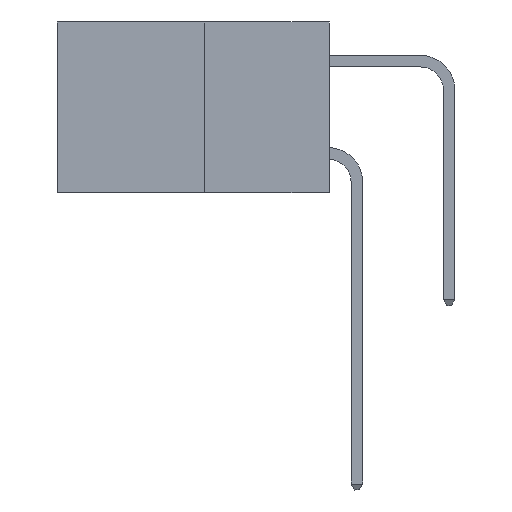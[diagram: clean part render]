
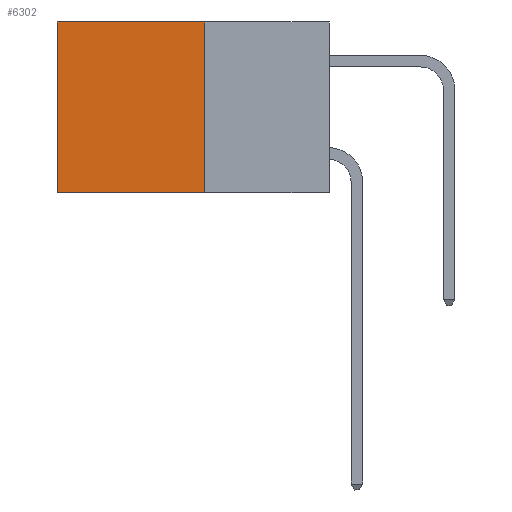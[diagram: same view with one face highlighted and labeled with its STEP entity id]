
A CAD part, left-side view. The second image highlights one B-rep face of the part: STEP entity #6302.
In plain terms, the highlighted planar face has unit normal (-1, 0, 0).
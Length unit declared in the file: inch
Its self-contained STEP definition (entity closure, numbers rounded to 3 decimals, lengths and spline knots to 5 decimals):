
#212 = CARTESIAN_POINT ( 'NONE',  ( 0.277, 0.27, -0.37 ) ) ;
#411 = DIRECTION ( 'NONE',  ( 0., 1., 0. ) ) ;
#683 = EDGE_LOOP ( 'NONE', ( #1466, #6687, #11780, #5957 ) ) ;
#749 = EDGE_CURVE ( 'NONE', #5637, #7984, #4505, .T. ) ;
#1007 = DIRECTION ( 'NONE',  ( 0., 0., -1. ) ) ;
#1109 = PLANE ( 'NONE',  #3783 ) ;
#1119 = EDGE_CURVE ( 'NONE', #7984, #6527, #11834, .T. ) ;
#1147 = DIRECTION ( 'NONE',  ( 1., 0., 0. ) ) ;
#1211 = DIRECTION ( 'NONE',  ( 0., 0., -1. ) ) ;
#1228 = CARTESIAN_POINT ( 'NONE',  ( 0.277, 0.27, -0.37 ) ) ;
#1466 = ORIENTED_EDGE ( 'NONE', *, *, #1119, .T. ) ;
#1794 = CARTESIAN_POINT ( 'NONE',  ( 0.277, 0.27, -0.37 ) ) ;
#1911 = DIRECTION ( 'NONE',  ( 0., 1., 0. ) ) ;
#2962 = CARTESIAN_POINT ( 'NONE',  ( 0.277, 0.27, 0. ) ) ;
#3019 = CARTESIAN_POINT ( 'NONE',  ( 0.277, 0.27, -0.37 ) ) ;
#3783 = AXIS2_PLACEMENT_3D ( 'NONE', #1794, #1147, #1007 ) ;
#4505 = LINE ( 'NONE', #8646, #9306 ) ;
#4783 = VECTOR ( 'NONE', #10424, 39.37008 ) ;
#5637 = VERTEX_POINT ( 'NONE', #2962 ) ;
#5957 = ORIENTED_EDGE ( 'NONE', *, *, #749, .T. ) ;
#5963 = EDGE_CURVE ( 'NONE', #8189, #6527, #12203, .T. ) ;
#6240 = FACE_OUTER_BOUND ( 'NONE', #683, .T. ) ;
#6280 = CARTESIAN_POINT ( 'NONE',  ( 0.277, 0.59, -0.37 ) ) ;
#6302 = ADVANCED_FACE ( 'NONE', ( #6240 ), #1109, .F. ) ;
#6527 = VERTEX_POINT ( 'NONE', #9547 ) ;
#6628 = CARTESIAN_POINT ( 'NONE',  ( 0.277, 0.59, 0. ) ) ;
#6687 = ORIENTED_EDGE ( 'NONE', *, *, #5963, .F. ) ;
#7213 = EDGE_CURVE ( 'NONE', #5637, #8189, #11351, .T. ) ;
#7984 = VERTEX_POINT ( 'NONE', #6628 ) ;
#8189 = VERTEX_POINT ( 'NONE', #3019 ) ;
#8646 = CARTESIAN_POINT ( 'NONE',  ( 0.277, 0.27, 0. ) ) ;
#8755 = VECTOR ( 'NONE', #1211, 39.37008 ) ;
#9306 = VECTOR ( 'NONE', #1911, 39.37008 ) ;
#9547 = CARTESIAN_POINT ( 'NONE',  ( 0.277, 0.59, -0.37 ) ) ;
#10424 = DIRECTION ( 'NONE',  ( 0., 0., -1. ) ) ;
#10531 = VECTOR ( 'NONE', #411, 39.37008 ) ;
#11351 = LINE ( 'NONE', #1228, #8755 ) ;
#11780 = ORIENTED_EDGE ( 'NONE', *, *, #7213, .F. ) ;
#11834 = LINE ( 'NONE', #6280, #4783 ) ;
#12203 = LINE ( 'NONE', #212, #10531 ) ;
